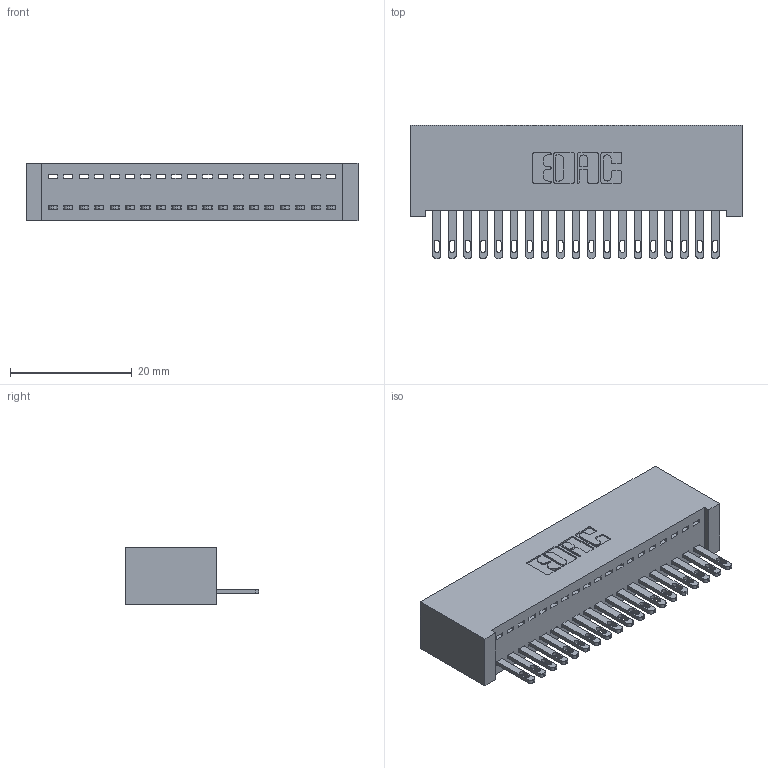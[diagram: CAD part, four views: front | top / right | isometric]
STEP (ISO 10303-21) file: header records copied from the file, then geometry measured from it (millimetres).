
FILE_DESCRIPTION (( 'STEP AP203' ), '1' );
FILE_NAME ('342-019-500-101.STEP', '2019-10-01T20:24:07', ( '' ), ( '' ), 'SwSTEP 2.0', 'SolidWorks 2016', '' );
FILE_SCHEMA (( 'CONFIG_CONTROL_DESIGN' ));
Length unit declared in the file: inch
Products named in the file (3): 342 Part_Lugless; 345-292-001_345-293-100; 342-019-500-101
Assembly tree (20 placements, depth 2):
  342-019-500-101
    342 Part_Lugless
    345-292-001_345-293-100  x19
Bounding box: 54.51 x 21.85 x 9.4 mm (x, y, z)
Volume: 5115.3 mm3; surface area: 7442.9 mm2
Topology: 20 solids, 20 shells, 1128 faces, 3467 edges, 2310 vertices
Faces by surface type: plane 746, cylinder 382
Entity records: 14111 total; most frequent: CARTESIAN_POINT 2443, ORIENTED_EDGE 2398, DIRECTION 2101, EDGE_CURVE 1199, VECTOR 1075, LINE 1075, VERTEX_POINT 798, AXIS2_PLACEMENT_3D 513
